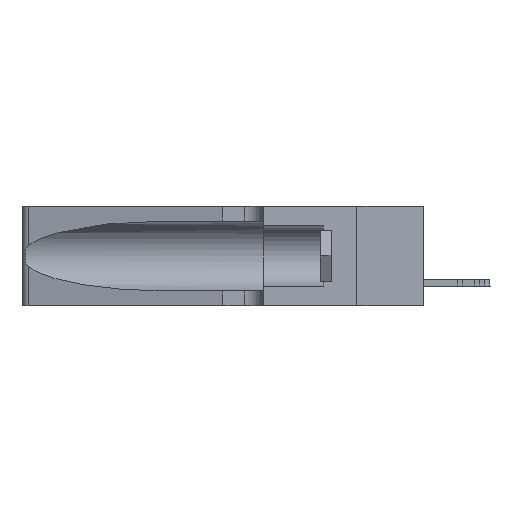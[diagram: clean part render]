
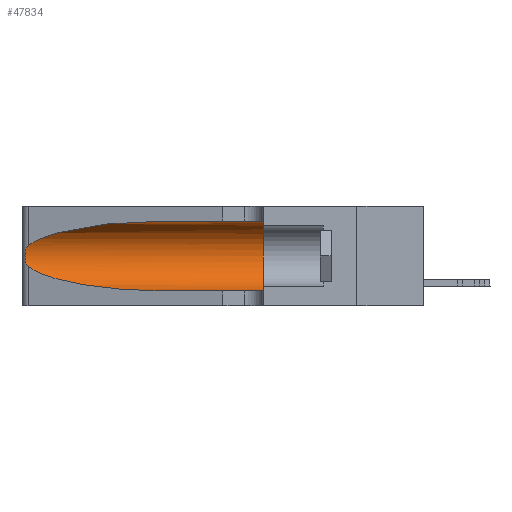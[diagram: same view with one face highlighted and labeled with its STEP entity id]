
A CAD part, left-side view. The second image highlights one B-rep face of the part: STEP entity #47834.
In plain terms, the highlighted cylindrical face has radius 3.308 mm (diameter 6.617 mm), a partial arc.
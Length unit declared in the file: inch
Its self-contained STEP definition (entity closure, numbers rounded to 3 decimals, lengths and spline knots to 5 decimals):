
#77 = ORIENTED_EDGE ( 'NONE', *, *, #41559, .T. ) ;
#548 = CARTESIAN_POINT ( 'NONE',  ( 0.1305, 0.72297, 0.05475 ) ) ;
#998 = CIRCLE ( 'NONE', #45794, 0.13025 ) ;
#1194 = CARTESIAN_POINT ( 'NONE',  ( 0.26017, 1.23833, 0.17102 ) ) ;
#1356 = CARTESIAN_POINT ( 'NONE',  ( 0.25555, 1.22993, 0.14849 ) ) ;
#2104 = ORIENTED_EDGE ( 'NONE', *, *, #45944, .T. ) ;
#2799 = CARTESIAN_POINT ( 'NONE',  ( 0.25487, 1.22718, 0.22369 ) ) ;
#6649 = CARTESIAN_POINT ( 'NONE',  ( 0.25639, 1.23184, 0.21858 ) ) ;
#8467 = EDGE_CURVE ( 'NONE', #18308, #33633, #14797, .T. ) ;
#8534 = CARTESIAN_POINT ( 'NONE',  ( 0.25639, 1.23186, 0.15144 ) ) ;
#8694 = DIRECTION ( 'NONE',  ( 0., -1., 0. ) ) ;
#9022 = CARTESIAN_POINT ( 'NONE',  ( 0.26075, 1.23896, 0.178 ) ) ;
#10810 = VERTEX_POINT ( 'NONE', #41119 ) ;
#13786 = DIRECTION ( 'NONE',  ( 0., -1., 0. ) ) ;
#14163 = AXIS2_PLACEMENT_3D ( 'NONE', #21684, #48510, #44549 ) ;
#14797 = LINE ( 'NONE', #34609, #26666 ) ;
#16487 = CARTESIAN_POINT ( 'NONE',  ( 0.25487, 1.22718, 0.14631 ) ) ;
#17998 = CARTESIAN_POINT ( 'NONE',  ( 0.2373, 1.15595, 0.28018 ) ) ;
#18017 = CYLINDRICAL_SURFACE ( 'NONE', #14163, 0.13025 ) ;
#18308 = VERTEX_POINT ( 'NONE', #25272 ) ;
#18845 = CARTESIAN_POINT ( 'NONE',  ( 0.1305, 0.35, 0.05475 ) ) ;
#21661 = EDGE_LOOP ( 'NONE', ( #47367, #34473, #77, #2104, #40893, #23483 ) ) ;
#21684 = CARTESIAN_POINT ( 'NONE',  ( 0.1305, 1.61858, 0.185 ) ) ;
#22811 = LINE ( 'NONE', #48271, #39312 ) ;
#23458 = CARTESIAN_POINT ( 'NONE',  ( 0.25856, 1.23593, 0.16098 ) ) ;
#23483 = ORIENTED_EDGE ( 'NONE', *, *, #8467, .F. ) ;
#25272 = CARTESIAN_POINT ( 'NONE',  ( 0.1305, 0.72297, 0.31525 ) ) ;
#25870 = CARTESIAN_POINT ( 'NONE',  ( 0.2373, 1.15595, 0.08982 ) ) ;
#26666 = VECTOR ( 'NONE', #8694, 39.37008 ) ;
#27764 = CARTESIAN_POINT ( 'NONE',  ( 0.1305, 0.35, 0.31525 ) ) ;
#27797 = VERTEX_POINT ( 'NONE', #548 ) ;
#28014 = EDGE_CURVE ( 'NONE', #18308, #46713, #40396, .T. ) ;
#29356 = CARTESIAN_POINT ( 'NONE',  ( 0.25555, 1.22994, 0.2215 ) ) ;
#29621 = CARTESIAN_POINT ( 'NONE',  ( 0.18966, 0.96281, 0.31525 ) ) ;
#29685 = CARTESIAN_POINT ( 'NONE',  ( 0.18966, 0.96281, 0.05475 ) ) ;
#31085 = EDGE_CURVE ( 'NONE', #46713, #10810, #31564, .T. ) ;
#31564 = B_SPLINE_CURVE_WITH_KNOTS ( 'NONE', 3,
 ( #2799, #29356, #6649, #40771, #43001, #38699, #42837, #9022, #1194, #23458, #39321, #8534, #1356, #16487 ),
 .UNSPECIFIED., .F., .F.,
 ( 4, 2, 2, 2, 2, 2, 4 ),
 ( 0., 0.00027, 0.00053, 0.00107, 0.0016, 0.00187, 0.00214 ),
 .UNSPECIFIED. ) ;
#31709 = CARTESIAN_POINT ( 'NONE',  ( 0.1305, 0.35, 0.185 ) ) ;
#33219 = EDGE_CURVE ( 'NONE', #33633, #34017, #998, .T. ) ;
#33509 = CARTESIAN_POINT ( 'NONE',  ( 0.1305, 0.72297, 0.05475 ) ) ;
#33633 = VERTEX_POINT ( 'NONE', #27764 ) ;
#33974 = CARTESIAN_POINT ( 'NONE',  ( 0.25487, 1.22718, 0.22369 ) ) ;
#34017 = VERTEX_POINT ( 'NONE', #18845 ) ;
#34473 = ORIENTED_EDGE ( 'NONE', *, *, #31085, .T. ) ;
#34609 = CARTESIAN_POINT ( 'NONE',  ( 0.1305, 1.61858, 0.31525 ) ) ;
#36800 = CARTESIAN_POINT ( 'NONE',  ( 0.25487, 1.22718, 0.14631 ) ) ;
#38699 = CARTESIAN_POINT ( 'NONE',  ( 0.26018, 1.23835, 0.19895 ) ) ;
#39312 = VECTOR ( 'NONE', #13786, 39.37008 ) ;
#39321 = CARTESIAN_POINT ( 'NONE',  ( 0.25789, 1.23486, 0.15765 ) ) ;
#40396 =( BOUNDED_CURVE ( )  B_SPLINE_CURVE ( 3, ( #46273, #29621, #17998, #40505 ),
 .UNSPECIFIED., .F., .F. ) 
 B_SPLINE_CURVE_WITH_KNOTS ( ( 4, 4 ),
 ( 1.5708, 2.84003 ),
 .UNSPECIFIED. ) 
 CURVE ( )  GEOMETRIC_REPRESENTATION_ITEM ( )  RATIONAL_B_SPLINE_CURVE ( ( 1., 0.87, 0.87, 1. ) ) 
 REPRESENTATION_ITEM ( '' )  );
#40505 = CARTESIAN_POINT ( 'NONE',  ( 0.25487, 1.22718, 0.22369 ) ) ;
#40771 = CARTESIAN_POINT ( 'NONE',  ( 0.25787, 1.23484, 0.2124 ) ) ;
#40893 = ORIENTED_EDGE ( 'NONE', *, *, #33219, .F. ) ;
#41119 = CARTESIAN_POINT ( 'NONE',  ( 0.25487, 1.22718, 0.14631 ) ) ;
#41559 = EDGE_CURVE ( 'NONE', #10810, #27797, #47884, .T. ) ;
#42837 = CARTESIAN_POINT ( 'NONE',  ( 0.26075, 1.23896, 0.19203 ) ) ;
#43001 = CARTESIAN_POINT ( 'NONE',  ( 0.25854, 1.2359, 0.20912 ) ) ;
#43449 = FACE_OUTER_BOUND ( 'NONE', #21661, .T. ) ;
#43675 = DIRECTION ( 'NONE',  ( 0., 1., 0. ) ) ;
#44549 = DIRECTION ( 'NONE',  ( 0., 0., -1. ) ) ;
#45794 = AXIS2_PLACEMENT_3D ( 'NONE', #31709, #43675, #48343 ) ;
#45944 = EDGE_CURVE ( 'NONE', #27797, #34017, #22811, .T. ) ;
#46273 = CARTESIAN_POINT ( 'NONE',  ( 0.1305, 0.72297, 0.31525 ) ) ;
#46713 = VERTEX_POINT ( 'NONE', #33974 ) ;
#47367 = ORIENTED_EDGE ( 'NONE', *, *, #28014, .T. ) ;
#47834 = ADVANCED_FACE ( 'NONE', ( #43449 ), #18017, .F. ) ;
#47884 =( BOUNDED_CURVE ( )  B_SPLINE_CURVE ( 3, ( #36800, #25870, #29685, #33509 ),
 .UNSPECIFIED., .F., .F. ) 
 B_SPLINE_CURVE_WITH_KNOTS ( ( 4, 4 ),
 ( 3.44316, 4.71239 ),
 .UNSPECIFIED. ) 
 CURVE ( )  GEOMETRIC_REPRESENTATION_ITEM ( )  RATIONAL_B_SPLINE_CURVE ( ( 1., 0.87, 0.87, 1. ) ) 
 REPRESENTATION_ITEM ( '' )  );
#48271 = CARTESIAN_POINT ( 'NONE',  ( 0.1305, 1.61858, 0.05475 ) ) ;
#48343 = DIRECTION ( 'NONE',  ( 0., 0., 1. ) ) ;
#48510 = DIRECTION ( 'NONE',  ( 0., -1., 0. ) ) ;
